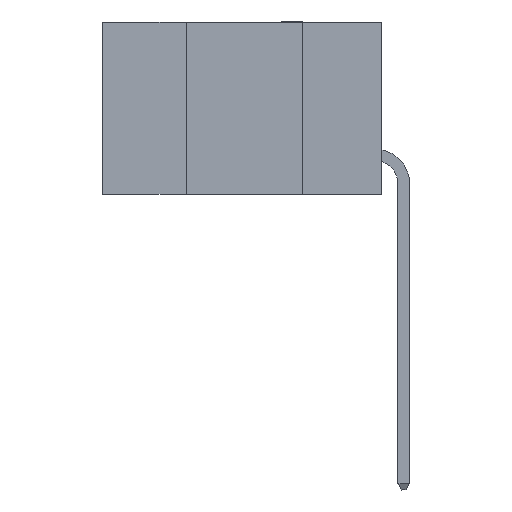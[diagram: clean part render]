
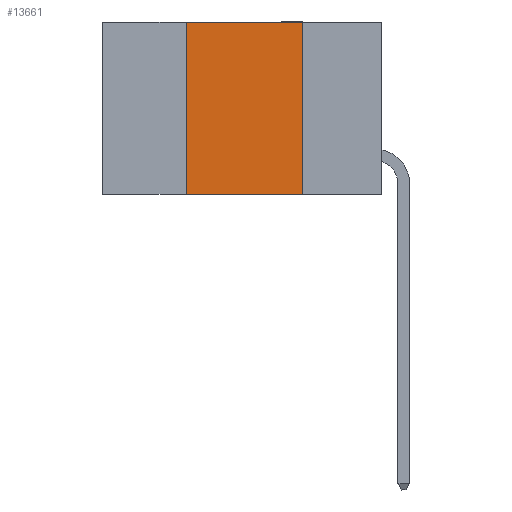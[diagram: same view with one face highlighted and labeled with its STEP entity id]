
A CAD part, left-side view. The second image highlights one B-rep face of the part: STEP entity #13661.
In plain terms, the highlighted planar face has unit normal (-1, 0, 0).
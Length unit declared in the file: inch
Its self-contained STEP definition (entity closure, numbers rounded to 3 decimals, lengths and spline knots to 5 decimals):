
#553 = VERTEX_POINT ( 'NONE', #10017 ) ;
#650 = EDGE_CURVE ( 'NONE', #9976, #1279, #8403, .T. ) ;
#878 = DIRECTION ( 'NONE',  ( 0., -1., 0. ) ) ;
#898 = DIRECTION ( 'NONE',  ( 1., 0., 0. ) ) ;
#1279 = VERTEX_POINT ( 'NONE', #10340 ) ;
#1530 = EDGE_CURVE ( 'NONE', #553, #6530, #2333, .T. ) ;
#2145 = CARTESIAN_POINT ( 'NONE',  ( 0., 0.6, 0. ) ) ;
#2333 = LINE ( 'NONE', #9259, #8368 ) ;
#3109 = CARTESIAN_POINT ( 'NONE',  ( 0., 0.17, -0.37 ) ) ;
#3556 = DIRECTION ( 'NONE',  ( 0., 0., -1. ) ) ;
#3626 = DIRECTION ( 'NONE',  ( 0., -1., 0. ) ) ;
#4443 = VECTOR ( 'NONE', #878, 39.37008 ) ;
#5456 = AXIS2_PLACEMENT_3D ( 'NONE', #2145, #898, #9857 ) ;
#5547 = DIRECTION ( 'NONE',  ( 0., 0., 1. ) ) ;
#5710 = ORIENTED_EDGE ( 'NONE', *, *, #16188, .T. ) ;
#6019 = PLANE ( 'NONE',  #5456 ) ;
#6530 = VERTEX_POINT ( 'NONE', #3109 ) ;
#7462 = CARTESIAN_POINT ( 'NONE',  ( 0., 0.6, -0.37 ) ) ;
#7885 = FACE_OUTER_BOUND ( 'NONE', #9273, .T. ) ;
#8368 = VECTOR ( 'NONE', #3556, 39.37008 ) ;
#8403 = LINE ( 'NONE', #13732, #15761 ) ;
#9259 = CARTESIAN_POINT ( 'NONE',  ( 0., 0.17, 0. ) ) ;
#9273 = EDGE_LOOP ( 'NONE', ( #13401, #10526, #12075, #5710 ) ) ;
#9857 = DIRECTION ( 'NONE',  ( 0., 0., -1. ) ) ;
#9976 = VERTEX_POINT ( 'NONE', #11738 ) ;
#10017 = CARTESIAN_POINT ( 'NONE',  ( 0., 0.17, 0. ) ) ;
#10261 = VECTOR ( 'NONE', #3626, 39.37008 ) ;
#10340 = CARTESIAN_POINT ( 'NONE',  ( 0., 0.42, 0. ) ) ;
#10526 = ORIENTED_EDGE ( 'NONE', *, *, #14303, .F. ) ;
#11260 = LINE ( 'NONE', #15990, #4443 ) ;
#11738 = CARTESIAN_POINT ( 'NONE',  ( 0., 0.42, -0.37 ) ) ;
#12075 = ORIENTED_EDGE ( 'NONE', *, *, #650, .F. ) ;
#13401 = ORIENTED_EDGE ( 'NONE', *, *, #1530, .F. ) ;
#13538 = LINE ( 'NONE', #7462, #10261 ) ;
#13661 = ADVANCED_FACE ( 'NONE', ( #7885 ), #6019, .F. ) ;
#13732 = CARTESIAN_POINT ( 'NONE',  ( 0., 0.42, 0. ) ) ;
#14303 = EDGE_CURVE ( 'NONE', #1279, #553, #11260, .T. ) ;
#15761 = VECTOR ( 'NONE', #5547, 39.37008 ) ;
#15990 = CARTESIAN_POINT ( 'NONE',  ( 0., 0.6, 0. ) ) ;
#16188 = EDGE_CURVE ( 'NONE', #9976, #6530, #13538, .T. ) ;
